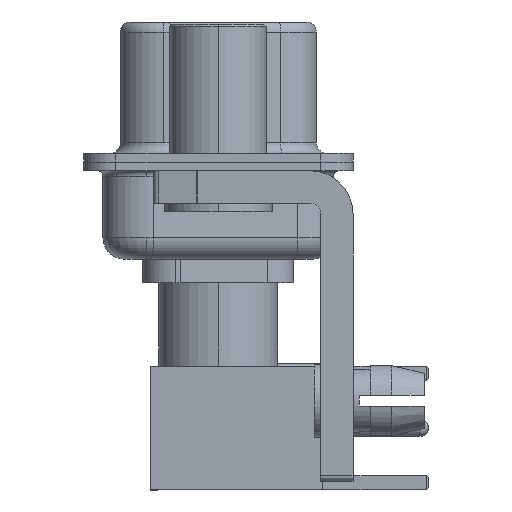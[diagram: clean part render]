
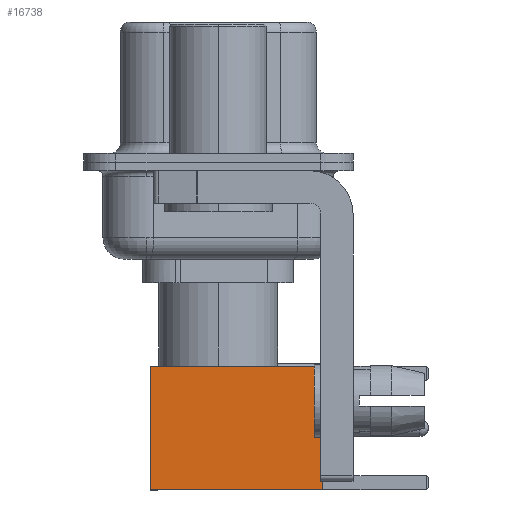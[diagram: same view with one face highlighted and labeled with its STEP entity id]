
A CAD part, left-side view. The second image highlights one B-rep face of the part: STEP entity #16738.
In plain terms, the highlighted face is planar.
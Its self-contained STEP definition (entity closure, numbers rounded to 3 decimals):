
#602 = EDGE_CURVE ( 'NONE', #8940, #13011, #29537, .T. ) ;
#2079 = DIRECTION ( 'NONE',  ( 0., 0., -1. ) ) ;
#2845 = VECTOR ( 'NONE', #31702, 1000. ) ;
#3364 = LINE ( 'NONE', #13423, #19177 ) ;
#3444 = EDGE_CURVE ( 'NONE', #22684, #24930, #14275, .T. ) ;
#4155 = DIRECTION ( 'NONE',  ( 0., 0., 1. ) ) ;
#4707 = CARTESIAN_POINT ( 'NONE',  ( -2.875, 2.875, 0. ) ) ;
#6098 = ORIENTED_EDGE ( 'NONE', *, *, #16224, .T. ) ;
#6592 = AXIS2_PLACEMENT_3D ( 'NONE', #14524, #31819, #4155 ) ;
#8940 = VERTEX_POINT ( 'NONE', #26184 ) ;
#9659 = ORIENTED_EDGE ( 'NONE', *, *, #3444, .F. ) ;
#10086 = CARTESIAN_POINT ( 'NONE',  ( 2.875, 2.875, 0. ) ) ;
#13011 = VERTEX_POINT ( 'NONE', #27583 ) ;
#13423 = CARTESIAN_POINT ( 'NONE',  ( 0., 2.875, 8. ) ) ;
#14087 = LINE ( 'NONE', #21646, #2845 ) ;
#14275 = LINE ( 'NONE', #4707, #17650 ) ;
#14524 = CARTESIAN_POINT ( 'NONE',  ( 2.875, 2.875, 0. ) ) ;
#15377 = ORIENTED_EDGE ( 'NONE', *, *, #16096, .F. ) ;
#15895 = CARTESIAN_POINT ( 'NONE',  ( -2.875, 2.875, 8. ) ) ;
#15941 = VECTOR ( 'NONE', #17503, 1000. ) ;
#16096 = EDGE_CURVE ( 'NONE', #8940, #22684, #3364, .T. ) ;
#16224 = EDGE_CURVE ( 'NONE', #13011, #24930, #14087, .T. ) ;
#16701 = ORIENTED_EDGE ( 'NONE', *, *, #602, .T. ) ;
#16738 = ADVANCED_FACE ( 'NONE', ( #19790 ), #19140, .T. ) ;
#17503 = DIRECTION ( 'NONE',  ( 0., 0., -1. ) ) ;
#17650 = VECTOR ( 'NONE', #2079, 1000. ) ;
#19140 = PLANE ( 'NONE',  #6592 ) ;
#19177 = VECTOR ( 'NONE', #23476, 1000. ) ;
#19790 = FACE_OUTER_BOUND ( 'NONE', #25668, .T. ) ;
#21646 = CARTESIAN_POINT ( 'NONE',  ( 0., 2.875, 0. ) ) ;
#22684 = VERTEX_POINT ( 'NONE', #15895 ) ;
#23476 = DIRECTION ( 'NONE',  ( -1., 0., 0. ) ) ;
#24657 = CARTESIAN_POINT ( 'NONE',  ( -2.875, 2.875, 0. ) ) ;
#24930 = VERTEX_POINT ( 'NONE', #24657 ) ;
#25668 = EDGE_LOOP ( 'NONE', ( #16701, #6098, #9659, #15377 ) ) ;
#26184 = CARTESIAN_POINT ( 'NONE',  ( 2.875, 2.875, 8. ) ) ;
#27583 = CARTESIAN_POINT ( 'NONE',  ( 2.875, 2.875, 0. ) ) ;
#29537 = LINE ( 'NONE', #10086, #15941 ) ;
#31702 = DIRECTION ( 'NONE',  ( -1., 0., 0. ) ) ;
#31819 = DIRECTION ( 'NONE',  ( 0., 1., 0. ) ) ;
